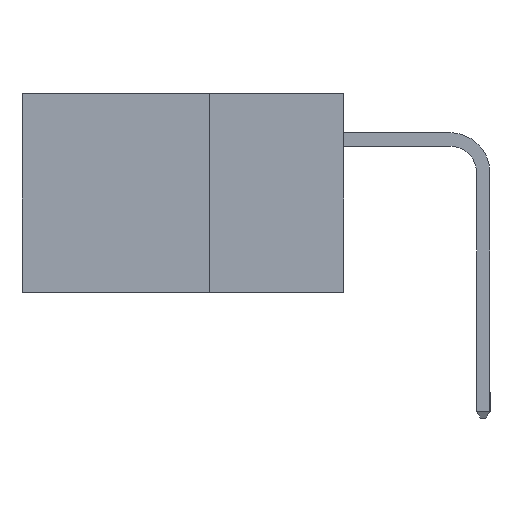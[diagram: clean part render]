
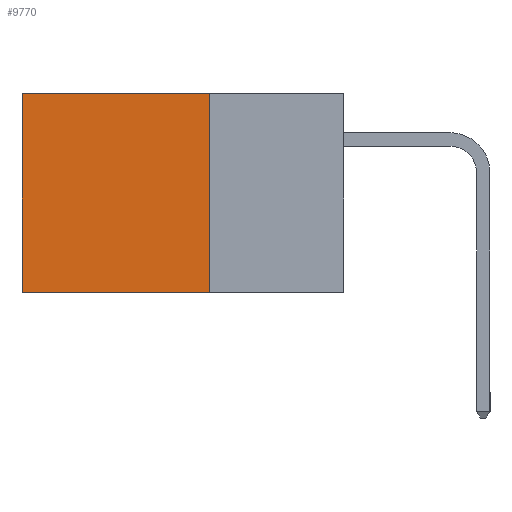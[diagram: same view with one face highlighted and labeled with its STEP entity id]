
A CAD part, left-side view. The second image highlights one B-rep face of the part: STEP entity #9770.
In plain terms, the highlighted planar face has unit normal (-1, 0, 0).
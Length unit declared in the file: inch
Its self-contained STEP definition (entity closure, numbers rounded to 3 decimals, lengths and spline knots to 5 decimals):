
#30 = EDGE_CURVE ( 'NONE', #4486, #5892, #9588, .T. ) ;
#63 = EDGE_CURVE ( 'NONE', #5892, #3980, #5309, .T. ) ;
#191 = CARTESIAN_POINT ( 'NONE',  ( 0.298, 0.25, 0. ) ) ;
#529 = FACE_OUTER_BOUND ( 'NONE', #1318, .T. ) ;
#1318 = EDGE_LOOP ( 'NONE', ( #3031, #12073, #10827, #1353 ) ) ;
#1353 = ORIENTED_EDGE ( 'NONE', *, *, #13439, .T. ) ;
#3031 = ORIENTED_EDGE ( 'NONE', *, *, #15734, .T. ) ;
#3980 = VERTEX_POINT ( 'NONE', #10729 ) ;
#4486 = VERTEX_POINT ( 'NONE', #4905 ) ;
#4621 = PLANE ( 'NONE',  #10902 ) ;
#4905 = CARTESIAN_POINT ( 'NONE',  ( 0.298, 0.25, 0. ) ) ;
#5309 = LINE ( 'NONE', #18015, #8230 ) ;
#5587 = DIRECTION ( 'NONE',  ( 0., 0., -1. ) ) ;
#5892 = VERTEX_POINT ( 'NONE', #13140 ) ;
#6034 = DIRECTION ( 'NONE',  ( 1., 0., 0. ) ) ;
#7662 = DIRECTION ( 'NONE',  ( 0., 1., 0. ) ) ;
#8230 = VECTOR ( 'NONE', #17495, 39.37008 ) ;
#9146 = VECTOR ( 'NONE', #16799, 39.37008 ) ;
#9588 = LINE ( 'NONE', #15794, #9146 ) ;
#9770 = ADVANCED_FACE ( 'NONE', ( #529 ), #4621, .F. ) ;
#9790 = LINE ( 'NONE', #17481, #13037 ) ;
#10453 = VERTEX_POINT ( 'NONE', #11783 ) ;
#10729 = CARTESIAN_POINT ( 'NONE',  ( 0.298, 0.6, -0.37 ) ) ;
#10827 = ORIENTED_EDGE ( 'NONE', *, *, #30, .F. ) ;
#10902 = AXIS2_PLACEMENT_3D ( 'NONE', #191, #6034, #15859 ) ;
#11783 = CARTESIAN_POINT ( 'NONE',  ( 0.298, 0.6, 0. ) ) ;
#12073 = ORIENTED_EDGE ( 'NONE', *, *, #63, .F. ) ;
#12973 = VECTOR ( 'NONE', #5587, 39.37008 ) ;
#13037 = VECTOR ( 'NONE', #7662, 39.37008 ) ;
#13140 = CARTESIAN_POINT ( 'NONE',  ( 0.298, 0.25, -0.37 ) ) ;
#13439 = EDGE_CURVE ( 'NONE', #4486, #10453, #9790, .T. ) ;
#15734 = EDGE_CURVE ( 'NONE', #10453, #3980, #16677, .T. ) ;
#15794 = CARTESIAN_POINT ( 'NONE',  ( 0.298, 0.25, 0. ) ) ;
#15859 = DIRECTION ( 'NONE',  ( 0., 0., -1. ) ) ;
#16677 = LINE ( 'NONE', #18205, #12973 ) ;
#16799 = DIRECTION ( 'NONE',  ( 0., 0., -1. ) ) ;
#17481 = CARTESIAN_POINT ( 'NONE',  ( 0.298, 0.25, 0. ) ) ;
#17495 = DIRECTION ( 'NONE',  ( 0., 1., 0. ) ) ;
#18015 = CARTESIAN_POINT ( 'NONE',  ( 0.298, 0.25, -0.37 ) ) ;
#18205 = CARTESIAN_POINT ( 'NONE',  ( 0.298, 0.6, 0. ) ) ;
